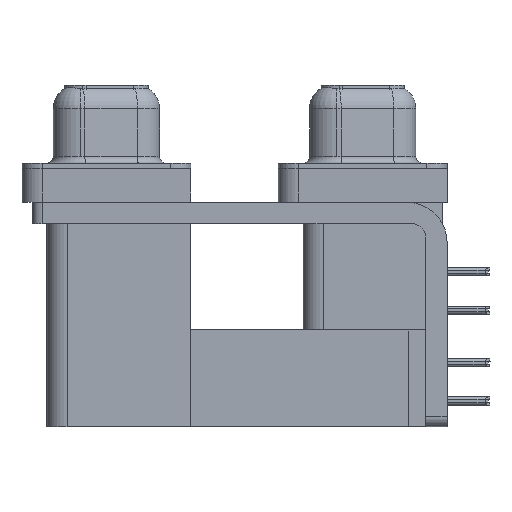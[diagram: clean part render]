
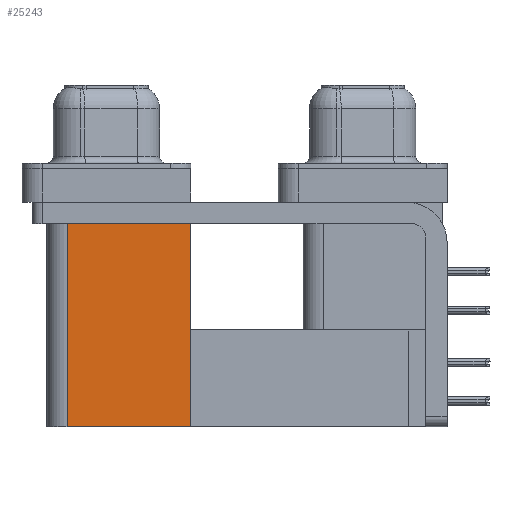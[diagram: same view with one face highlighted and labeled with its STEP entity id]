
A CAD part, left-side view. The second image highlights one B-rep face of the part: STEP entity #25243.
In plain terms, the highlighted planar face has unit normal (-1, 0, 0).
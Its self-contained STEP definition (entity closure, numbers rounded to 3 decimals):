
#481 = EDGE_CURVE ( 'NONE', #22945, #31961, #7490, .T. ) ;
#1350 = PLANE ( 'NONE',  #14056 ) ;
#2161 = CARTESIAN_POINT ( 'NONE',  ( 3.765, 21.975, -2.5 ) ) ;
#4630 = ORIENTED_EDGE ( 'NONE', *, *, #481, .F. ) ;
#4835 = DIRECTION ( 'NONE',  ( 0., 0., -1. ) ) ;
#5317 = FACE_OUTER_BOUND ( 'NONE', #24406, .T. ) ;
#6627 = ORIENTED_EDGE ( 'NONE', *, *, #39763, .T. ) ;
#7490 = LINE ( 'NONE', #22532, #36075 ) ;
#9905 = EDGE_CURVE ( 'NONE', #10593, #23979, #47780, .T. ) ;
#10593 = VERTEX_POINT ( 'NONE', #27156 ) ;
#13190 = LINE ( 'NONE', #35188, #25463 ) ;
#14056 = AXIS2_PLACEMENT_3D ( 'NONE', #27061, #34481, #4835 ) ;
#16846 = ORIENTED_EDGE ( 'NONE', *, *, #45883, .F. ) ;
#17834 = CARTESIAN_POINT ( 'NONE',  ( 3.765, 21.975, -19.2 ) ) ;
#18826 = DIRECTION ( 'NONE',  ( 0., 0., 1. ) ) ;
#19531 = CARTESIAN_POINT ( 'NONE',  ( 3.765, 12.775, -19.2 ) ) ;
#22532 = CARTESIAN_POINT ( 'NONE',  ( 3.765, 21.975, -19.2 ) ) ;
#22945 = VERTEX_POINT ( 'NONE', #17834 ) ;
#23979 = VERTEX_POINT ( 'NONE', #29930 ) ;
#24406 = EDGE_LOOP ( 'NONE', ( #6627, #4630, #16846, #30314 ) ) ;
#24785 = CARTESIAN_POINT ( 'NONE',  ( 3.765, 12.775, -19.2 ) ) ;
#25243 = ADVANCED_FACE ( 'NONE', ( #5317 ), #1350, .F. ) ;
#25463 = VECTOR ( 'NONE', #28251, 1000. ) ;
#25623 = VECTOR ( 'NONE', #25748, 1000. ) ;
#25748 = DIRECTION ( 'NONE',  ( 0., 0., 1. ) ) ;
#26478 = LINE ( 'NONE', #19531, #36762 ) ;
#27061 = CARTESIAN_POINT ( 'NONE',  ( 3.765, 12.775, -19.2 ) ) ;
#27156 = CARTESIAN_POINT ( 'NONE',  ( 3.765, 12.775, -19.2 ) ) ;
#28251 = DIRECTION ( 'NONE',  ( 0., 1., 0. ) ) ;
#29930 = CARTESIAN_POINT ( 'NONE',  ( 3.765, 12.775, -2.5 ) ) ;
#30314 = ORIENTED_EDGE ( 'NONE', *, *, #9905, .T. ) ;
#31961 = VERTEX_POINT ( 'NONE', #2161 ) ;
#34481 = DIRECTION ( 'NONE',  ( 1., 0., 0. ) ) ;
#35188 = CARTESIAN_POINT ( 'NONE',  ( 3.765, 12.775, -2.5 ) ) ;
#36075 = VECTOR ( 'NONE', #18826, 1000. ) ;
#36762 = VECTOR ( 'NONE', #45500, 1000. ) ;
#39763 = EDGE_CURVE ( 'NONE', #23979, #31961, #13190, .T. ) ;
#45500 = DIRECTION ( 'NONE',  ( 0., 1., 0. ) ) ;
#45883 = EDGE_CURVE ( 'NONE', #10593, #22945, #26478, .T. ) ;
#47780 = LINE ( 'NONE', #24785, #25623 ) ;
